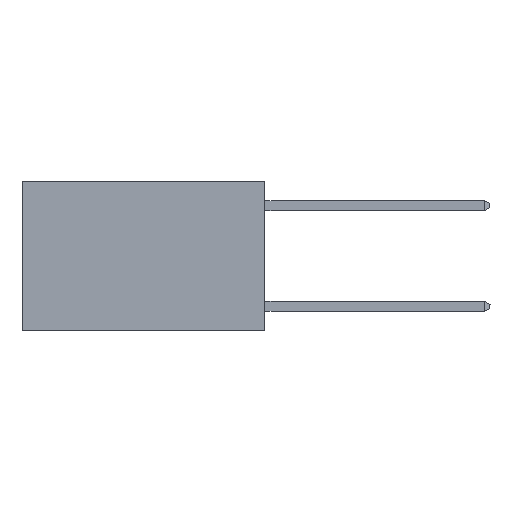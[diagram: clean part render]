
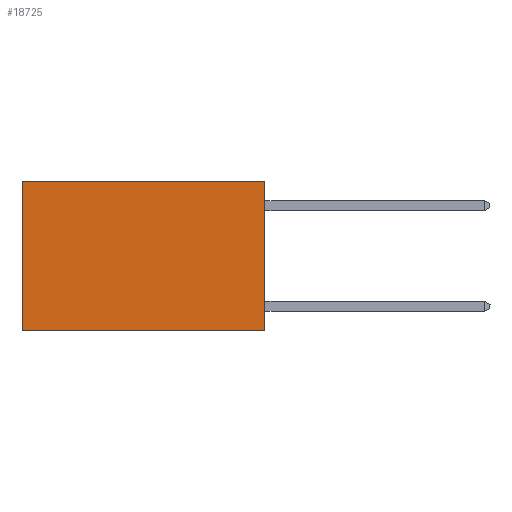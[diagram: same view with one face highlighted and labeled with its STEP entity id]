
A CAD part, left-side view. The second image highlights one B-rep face of the part: STEP entity #18725.
In plain terms, the highlighted planar face has unit normal (-1, 0, 0).
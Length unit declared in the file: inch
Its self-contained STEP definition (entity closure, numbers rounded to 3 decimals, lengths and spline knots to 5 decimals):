
#786 = DIRECTION ( 'NONE',  ( 0., 0., -1. ) ) ;
#1122 = DIRECTION ( 'NONE',  ( 0., 1., 0. ) ) ;
#1233 = VERTEX_POINT ( 'NONE', #19112 ) ;
#1426 = VECTOR ( 'NONE', #12051, 39.37008 ) ;
#2269 = VECTOR ( 'NONE', #786, 39.37008 ) ;
#2517 = EDGE_CURVE ( 'NONE', #16466, #18604, #19894, .T. ) ;
#2538 = ORIENTED_EDGE ( 'NONE', *, *, #2517, .T. ) ;
#3876 = CARTESIAN_POINT ( 'NONE',  ( 0.2625, 0., -0.37 ) ) ;
#3911 = EDGE_CURVE ( 'NONE', #16466, #19513, #5154, .T. ) ;
#5154 = LINE ( 'NONE', #16879, #6119 ) ;
#5457 = CARTESIAN_POINT ( 'NONE',  ( 0.2625, 0., -0.37 ) ) ;
#6119 = VECTOR ( 'NONE', #18606, 39.37008 ) ;
#8130 = PLANE ( 'NONE',  #17504 ) ;
#8385 = EDGE_CURVE ( 'NONE', #18604, #1233, #15742, .T. ) ;
#9085 = VECTOR ( 'NONE', #1122, 39.37008 ) ;
#9677 = DIRECTION ( 'NONE',  ( 0., 0., -1. ) ) ;
#10304 = CARTESIAN_POINT ( 'NONE',  ( 0.2625, 0., 0. ) ) ;
#10875 = CARTESIAN_POINT ( 'NONE',  ( 0.2625, 0.6, 0. ) ) ;
#11019 = DIRECTION ( 'NONE',  ( 1., 0., 0. ) ) ;
#11465 = FACE_OUTER_BOUND ( 'NONE', #11858, .T. ) ;
#11858 = EDGE_LOOP ( 'NONE', ( #19889, #15282, #16979, #2538 ) ) ;
#12051 = DIRECTION ( 'NONE',  ( 0., 1., 0. ) ) ;
#14578 = CARTESIAN_POINT ( 'NONE',  ( 0.2625, 0.6, 0. ) ) ;
#14620 = CARTESIAN_POINT ( 'NONE',  ( 0.2625, 0., 0. ) ) ;
#15282 = ORIENTED_EDGE ( 'NONE', *, *, #16766, .F. ) ;
#15742 = LINE ( 'NONE', #14578, #2269 ) ;
#16092 = LINE ( 'NONE', #5457, #1426 ) ;
#16466 = VERTEX_POINT ( 'NONE', #14620 ) ;
#16766 = EDGE_CURVE ( 'NONE', #19513, #1233, #16092, .T. ) ;
#16879 = CARTESIAN_POINT ( 'NONE',  ( 0.2625, 0., 0. ) ) ;
#16979 = ORIENTED_EDGE ( 'NONE', *, *, #3911, .F. ) ;
#17149 = CARTESIAN_POINT ( 'NONE',  ( 0.2625, 0., 0. ) ) ;
#17504 = AXIS2_PLACEMENT_3D ( 'NONE', #17149, #11019, #9677 ) ;
#18604 = VERTEX_POINT ( 'NONE', #10875 ) ;
#18606 = DIRECTION ( 'NONE',  ( 0., 0., -1. ) ) ;
#18725 = ADVANCED_FACE ( 'NONE', ( #11465 ), #8130, .F. ) ;
#19112 = CARTESIAN_POINT ( 'NONE',  ( 0.2625, 0.6, -0.37 ) ) ;
#19513 = VERTEX_POINT ( 'NONE', #3876 ) ;
#19889 = ORIENTED_EDGE ( 'NONE', *, *, #8385, .T. ) ;
#19894 = LINE ( 'NONE', #10304, #9085 ) ;
